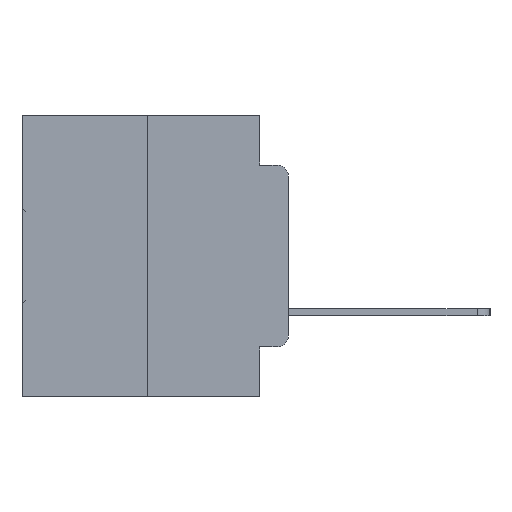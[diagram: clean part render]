
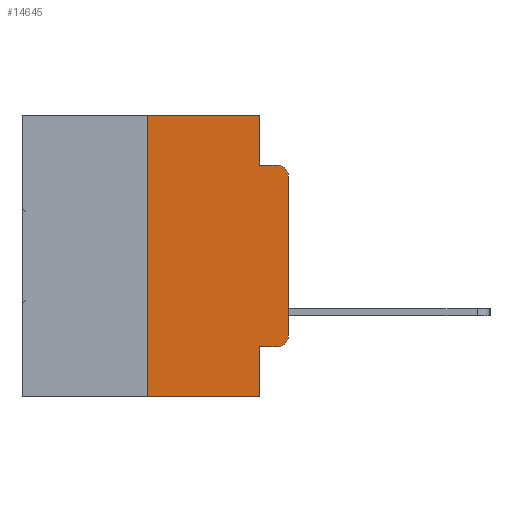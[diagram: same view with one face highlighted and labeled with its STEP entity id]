
A CAD part, left-side view. The second image highlights one B-rep face of the part: STEP entity #14645.
In plain terms, the highlighted planar face has unit normal (-1, 0, 0).
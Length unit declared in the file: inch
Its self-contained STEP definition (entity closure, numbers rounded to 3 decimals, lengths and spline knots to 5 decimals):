
#353 = EDGE_CURVE ( 'NONE', #31235, #30583, #3188, .T. ) ;
#968 = VERTEX_POINT ( 'NONE', #9433 ) ;
#1020 = EDGE_CURVE ( 'NONE', #21171, #12135, #25617, .T. ) ;
#1532 = DIRECTION ( 'NONE',  ( 0., 0., 1. ) ) ;
#1875 = CARTESIAN_POINT ( 'NONE',  ( 0., 0.051, -0.0885 ) ) ;
#2137 = EDGE_CURVE ( 'NONE', #968, #31235, #4609, .T. ) ;
#2203 = LINE ( 'NONE', #28477, #21001 ) ;
#2213 = PLANE ( 'NONE',  #13702 ) ;
#2222 = DIRECTION ( 'NONE',  ( 0., 0., -1. ) ) ;
#2645 = EDGE_CURVE ( 'NONE', #9100, #8496, #2203, .T. ) ;
#2894 = CARTESIAN_POINT ( 'NONE',  ( 0., 0.051, 0. ) ) ;
#3188 = CIRCLE ( 'NONE', #5539, 0.02 ) ;
#3282 = LINE ( 'NONE', #15846, #9092 ) ;
#3651 = LINE ( 'NONE', #21920, #8704 ) ;
#4129 = CARTESIAN_POINT ( 'NONE',  ( 0., 0.02, -0.3915 ) ) ;
#4253 = VECTOR ( 'NONE', #2222, 39.37008 ) ;
#4609 = LINE ( 'NONE', #6400, #29578 ) ;
#5408 = CARTESIAN_POINT ( 'NONE',  ( 0., 0.02, -0.1085 ) ) ;
#5539 = AXIS2_PLACEMENT_3D ( 'NONE', #5408, #13155, #15426 ) ;
#6400 = CARTESIAN_POINT ( 'NONE',  ( 0., 0., 0. ) ) ;
#6638 = DIRECTION ( 'NONE',  ( 0., 0., -1. ) ) ;
#7256 = DIRECTION ( 'NONE',  ( 1., 0., 0. ) ) ;
#7367 = DIRECTION ( 'NONE',  ( 0., -1., 0. ) ) ;
#7816 = CARTESIAN_POINT ( 'NONE',  ( 0., 0.02, -0.0885 ) ) ;
#8325 = VECTOR ( 'NONE', #12151, 39.37008 ) ;
#8496 = VERTEX_POINT ( 'NONE', #9730 ) ;
#8704 = VECTOR ( 'NONE', #7367, 39.37008 ) ;
#9092 = VECTOR ( 'NONE', #1532, 39.37008 ) ;
#9100 = VERTEX_POINT ( 'NONE', #12185 ) ;
#9433 = CARTESIAN_POINT ( 'NONE',  ( 0., 0., -0.3915 ) ) ;
#9660 = CARTESIAN_POINT ( 'NONE',  ( 0., 0.051, -0.0885 ) ) ;
#9730 = CARTESIAN_POINT ( 'NONE',  ( 0., 0.051, 0. ) ) ;
#10401 = CARTESIAN_POINT ( 'NONE',  ( 0., 0.051, -0.5 ) ) ;
#10871 = CARTESIAN_POINT ( 'NONE',  ( 0., 0.02, -0.4115 ) ) ;
#12135 = VERTEX_POINT ( 'NONE', #10871 ) ;
#12151 = DIRECTION ( 'NONE',  ( 0., -1., 0. ) ) ;
#12185 = CARTESIAN_POINT ( 'NONE',  ( 0., 0.25, 0. ) ) ;
#12392 = FACE_OUTER_BOUND ( 'NONE', #28717, .T. ) ;
#12505 = CIRCLE ( 'NONE', #25145, 0.02 ) ;
#12822 = VECTOR ( 'NONE', #25513, 39.37008 ) ;
#13155 = DIRECTION ( 'NONE',  ( -1., 0., 0. ) ) ;
#13702 = AXIS2_PLACEMENT_3D ( 'NONE', #16991, #7256, #24221 ) ;
#13732 = ORIENTED_EDGE ( 'NONE', *, *, #2137, .T. ) ;
#13834 = ORIENTED_EDGE ( 'NONE', *, *, #353, .T. ) ;
#13919 = ORIENTED_EDGE ( 'NONE', *, *, #28807, .F. ) ;
#14006 = ORIENTED_EDGE ( 'NONE', *, *, #25644, .F. ) ;
#14275 = ORIENTED_EDGE ( 'NONE', *, *, #2645, .F. ) ;
#14391 = ORIENTED_EDGE ( 'NONE', *, *, #24052, .F. ) ;
#14601 = VERTEX_POINT ( 'NONE', #1875 ) ;
#14619 = ORIENTED_EDGE ( 'NONE', *, *, #24295, .T. ) ;
#14645 = ADVANCED_FACE ( 'NONE', ( #12392 ), #2213, .F. ) ;
#14653 = ORIENTED_EDGE ( 'NONE', *, *, #17643, .F. ) ;
#15160 = ORIENTED_EDGE ( 'NONE', *, *, #1020, .T. ) ;
#15414 = ORIENTED_EDGE ( 'NONE', *, *, #29387, .T. ) ;
#15426 = DIRECTION ( 'NONE',  ( 0., 0., -1. ) ) ;
#15606 = LINE ( 'NONE', #9660, #8325 ) ;
#15764 = VECTOR ( 'NONE', #29601, 39.37008 ) ;
#15846 = CARTESIAN_POINT ( 'NONE',  ( 0., 0.25, 0. ) ) ;
#16323 = DIRECTION ( 'NONE',  ( 0., 0., 1. ) ) ;
#16991 = CARTESIAN_POINT ( 'NONE',  ( 0., 0.473, 0. ) ) ;
#17000 = CARTESIAN_POINT ( 'NONE',  ( 0., 0.051, 0. ) ) ;
#17643 = EDGE_CURVE ( 'NONE', #21171, #24958, #22954, .T. ) ;
#21001 = VECTOR ( 'NONE', #26657, 39.37008 ) ;
#21171 = VERTEX_POINT ( 'NONE', #29281 ) ;
#21227 = DIRECTION ( 'NONE',  ( -1., 0., 0. ) ) ;
#21766 = CARTESIAN_POINT ( 'NONE',  ( 0., 0.051, -0.4115 ) ) ;
#21920 = CARTESIAN_POINT ( 'NONE',  ( 0., 0.473, -0.5 ) ) ;
#22907 = LINE ( 'NONE', #2894, #15764 ) ;
#22954 = LINE ( 'NONE', #17000, #4253 ) ;
#23269 = CARTESIAN_POINT ( 'NONE',  ( 0., 0., -0.1085 ) ) ;
#24052 = EDGE_CURVE ( 'NONE', #26524, #9100, #3282, .T. ) ;
#24221 = DIRECTION ( 'NONE',  ( 0., 0., -1. ) ) ;
#24295 = EDGE_CURVE ( 'NONE', #26524, #24958, #3651, .T. ) ;
#24958 = VERTEX_POINT ( 'NONE', #10401 ) ;
#25145 = AXIS2_PLACEMENT_3D ( 'NONE', #4129, #21227, #6638 ) ;
#25513 = DIRECTION ( 'NONE',  ( 0., -1., 0. ) ) ;
#25617 = LINE ( 'NONE', #21766, #12822 ) ;
#25644 = EDGE_CURVE ( 'NONE', #8496, #14601, #22907, .T. ) ;
#26524 = VERTEX_POINT ( 'NONE', #28697 ) ;
#26657 = DIRECTION ( 'NONE',  ( 0., -1., 0. ) ) ;
#28477 = CARTESIAN_POINT ( 'NONE',  ( 0., 0.473, 0. ) ) ;
#28697 = CARTESIAN_POINT ( 'NONE',  ( 0., 0.25, -0.5 ) ) ;
#28717 = EDGE_LOOP ( 'NONE', ( #13732, #13834, #13919, #14006, #14275, #14391, #14619, #14653, #15160, #15414 ) ) ;
#28807 = EDGE_CURVE ( 'NONE', #14601, #30583, #15606, .T. ) ;
#29281 = CARTESIAN_POINT ( 'NONE',  ( 0., 0.051, -0.4115 ) ) ;
#29387 = EDGE_CURVE ( 'NONE', #12135, #968, #12505, .T. ) ;
#29578 = VECTOR ( 'NONE', #16323, 39.37008 ) ;
#29601 = DIRECTION ( 'NONE',  ( 0., 0., -1. ) ) ;
#30583 = VERTEX_POINT ( 'NONE', #7816 ) ;
#31235 = VERTEX_POINT ( 'NONE', #23269 ) ;
